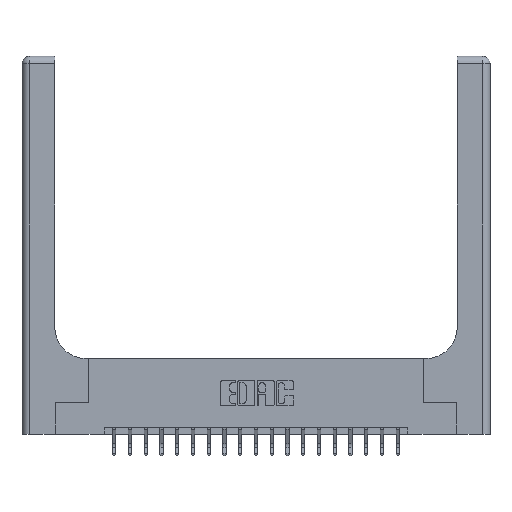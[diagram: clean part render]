
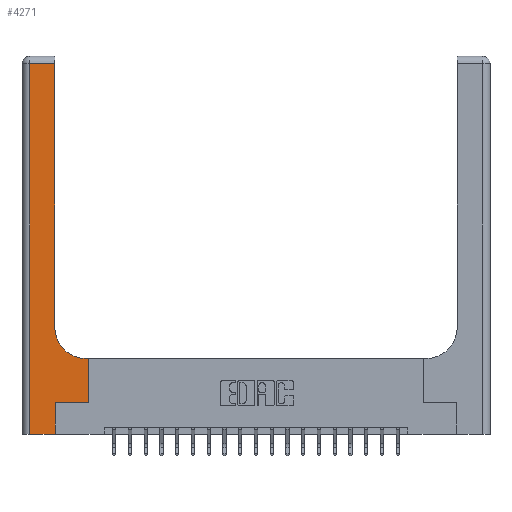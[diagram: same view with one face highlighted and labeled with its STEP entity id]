
A CAD part, top view. The second image highlights one B-rep face of the part: STEP entity #4271.
In plain terms, the highlighted planar face has unit normal (0, 0, 1).
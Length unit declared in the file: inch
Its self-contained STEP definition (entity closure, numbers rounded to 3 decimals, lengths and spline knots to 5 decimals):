
#93 = ORIENTED_EDGE ( 'NONE', *, *, #18552, .T. ) ;
#365 = CARTESIAN_POINT ( 'NONE',  ( 0.528, 0.6, 0.37 ) ) ;
#375 = AXIS2_PLACEMENT_3D ( 'NONE', #12498, #6096, #17427 ) ;
#439 = CARTESIAN_POINT ( 'NONE',  ( 0.26, 0.85, 0.37 ) ) ;
#460 = LINE ( 'NONE', #2405, #5534 ) ;
#911 = CARTESIAN_POINT ( 'NONE',  ( 0.26, 3., 0.37 ) ) ;
#1702 = LINE ( 'NONE', #12467, #7505 ) ;
#2405 = CARTESIAN_POINT ( 'NONE',  ( 0.528, 0.25, 0.37 ) ) ;
#2840 = CARTESIAN_POINT ( 'NONE',  ( 0.265, 0.25, 0.37 ) ) ;
#3224 = CARTESIAN_POINT ( 'NONE',  ( 0.265, 0., 0.37 ) ) ;
#3311 = VECTOR ( 'NONE', #4429, 39.37008 ) ;
#3415 = VECTOR ( 'NONE', #18501, 39.37008 ) ;
#3792 = VERTEX_POINT ( 'NONE', #15043 ) ;
#4210 = EDGE_CURVE ( 'NONE', #10183, #20117, #15230, .T. ) ;
#4271 = ADVANCED_FACE ( 'NONE', ( #19539 ), #18977, .F. ) ;
#4302 = EDGE_CURVE ( 'NONE', #5906, #20108, #9877, .T. ) ;
#4429 = DIRECTION ( 'NONE',  ( 0., 1., 0. ) ) ;
#4616 = EDGE_CURVE ( 'NONE', #3792, #16907, #8841, .T. ) ;
#4925 = ORIENTED_EDGE ( 'NONE', *, *, #9679, .T. ) ;
#5188 = EDGE_LOOP ( 'NONE', ( #9964, #17416, #14029, #93, #18827, #12260, #16908, #16149, #4925 ) ) ;
#5436 = VERTEX_POINT ( 'NONE', #3224 ) ;
#5534 = VECTOR ( 'NONE', #16976, 39.37008 ) ;
#5592 = CARTESIAN_POINT ( 'NONE',  ( 0.265, 0., 0.37 ) ) ;
#5887 = AXIS2_PLACEMENT_3D ( 'NONE', #16774, #13375, #19834 ) ;
#5906 = VERTEX_POINT ( 'NONE', #365 ) ;
#6087 = EDGE_CURVE ( 'NONE', #11094, #18965, #16161, .T. ) ;
#6096 = DIRECTION ( 'NONE',  ( 0., 0., -1. ) ) ;
#7355 = DIRECTION ( 'NONE',  ( 1., 0., 0. ) ) ;
#7505 = VECTOR ( 'NONE', #10619, 39.37008 ) ;
#7756 = CARTESIAN_POINT ( 'NONE',  ( 0.528, 0.25, 0.37 ) ) ;
#7861 = VECTOR ( 'NONE', #17200, 39.37008 ) ;
#8200 = CARTESIAN_POINT ( 'NONE',  ( 0.06, 3., 0.37 ) ) ;
#8841 = LINE ( 'NONE', #8200, #18525 ) ;
#9337 = EDGE_CURVE ( 'NONE', #5436, #11094, #12937, .T. ) ;
#9466 = CARTESIAN_POINT ( 'NONE',  ( 0.265, 0.25, 0.37 ) ) ;
#9679 = EDGE_CURVE ( 'NONE', #20108, #10183, #15219, .T. ) ;
#9877 = LINE ( 'NONE', #16404, #20787 ) ;
#9964 = ORIENTED_EDGE ( 'NONE', *, *, #4210, .T. ) ;
#10183 = VERTEX_POINT ( 'NONE', #439 ) ;
#10619 = DIRECTION ( 'NONE',  ( -1., 0., 0. ) ) ;
#11000 = LINE ( 'NONE', #13429, #3415 ) ;
#11094 = VERTEX_POINT ( 'NONE', #9466 ) ;
#11607 = CARTESIAN_POINT ( 'NONE',  ( 0.26, 2.94, 0.37 ) ) ;
#11820 = VECTOR ( 'NONE', #7355, 39.37008 ) ;
#12260 = ORIENTED_EDGE ( 'NONE', *, *, #6087, .T. ) ;
#12467 = CARTESIAN_POINT ( 'NONE',  ( 0., 2.94, 0.37 ) ) ;
#12498 = CARTESIAN_POINT ( 'NONE',  ( 0., 3., 0.37 ) ) ;
#12937 = LINE ( 'NONE', #5592, #3311 ) ;
#13375 = DIRECTION ( 'NONE',  ( 0., 0., -1. ) ) ;
#13429 = CARTESIAN_POINT ( 'NONE',  ( 0., 0., 0.37 ) ) ;
#14029 = ORIENTED_EDGE ( 'NONE', *, *, #4616, .T. ) ;
#15043 = CARTESIAN_POINT ( 'NONE',  ( 0.06, 2.94, 0.37 ) ) ;
#15219 = CIRCLE ( 'NONE', #5887, 0.25 ) ;
#15230 = LINE ( 'NONE', #911, #7861 ) ;
#15670 = CARTESIAN_POINT ( 'NONE',  ( 0.51, 0.6, 0.37 ) ) ;
#16149 = ORIENTED_EDGE ( 'NONE', *, *, #4302, .T. ) ;
#16161 = LINE ( 'NONE', #2840, #11820 ) ;
#16404 = CARTESIAN_POINT ( 'NONE',  ( 0.26, 0.6, 0.37 ) ) ;
#16445 = DIRECTION ( 'NONE',  ( 0., -1., 0. ) ) ;
#16651 = EDGE_CURVE ( 'NONE', #18965, #5906, #460, .T. ) ;
#16774 = CARTESIAN_POINT ( 'NONE',  ( 0.51, 0.85, 0.37 ) ) ;
#16907 = VERTEX_POINT ( 'NONE', #20123 ) ;
#16908 = ORIENTED_EDGE ( 'NONE', *, *, #16651, .T. ) ;
#16976 = DIRECTION ( 'NONE',  ( 0., 1., 0. ) ) ;
#17016 = EDGE_CURVE ( 'NONE', #20117, #3792, #1702, .T. ) ;
#17200 = DIRECTION ( 'NONE',  ( 0., 1., 0. ) ) ;
#17416 = ORIENTED_EDGE ( 'NONE', *, *, #17016, .T. ) ;
#17427 = DIRECTION ( 'NONE',  ( -1., 0., 0. ) ) ;
#18501 = DIRECTION ( 'NONE',  ( 1., 0., 0. ) ) ;
#18525 = VECTOR ( 'NONE', #16445, 39.37008 ) ;
#18552 = EDGE_CURVE ( 'NONE', #16907, #5436, #11000, .T. ) ;
#18827 = ORIENTED_EDGE ( 'NONE', *, *, #9337, .T. ) ;
#18965 = VERTEX_POINT ( 'NONE', #7756 ) ;
#18977 = PLANE ( 'NONE',  #375 ) ;
#19539 = FACE_OUTER_BOUND ( 'NONE', #5188, .T. ) ;
#19661 = DIRECTION ( 'NONE',  ( -1., 0., 0. ) ) ;
#19834 = DIRECTION ( 'NONE',  ( 1., 0., 0. ) ) ;
#20108 = VERTEX_POINT ( 'NONE', #15670 ) ;
#20117 = VERTEX_POINT ( 'NONE', #11607 ) ;
#20123 = CARTESIAN_POINT ( 'NONE',  ( 0.06, 0., 0.37 ) ) ;
#20787 = VECTOR ( 'NONE', #19661, 39.37008 ) ;
